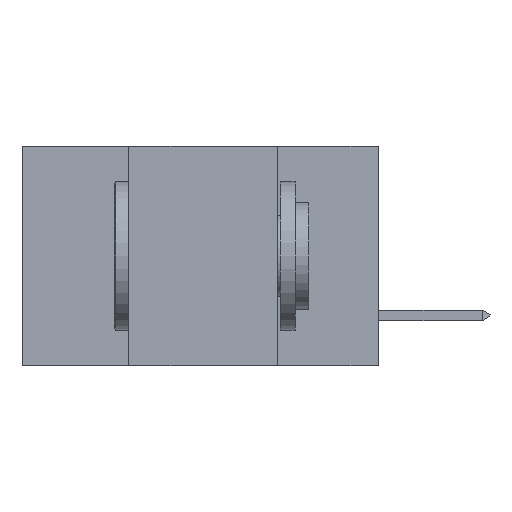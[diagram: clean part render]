
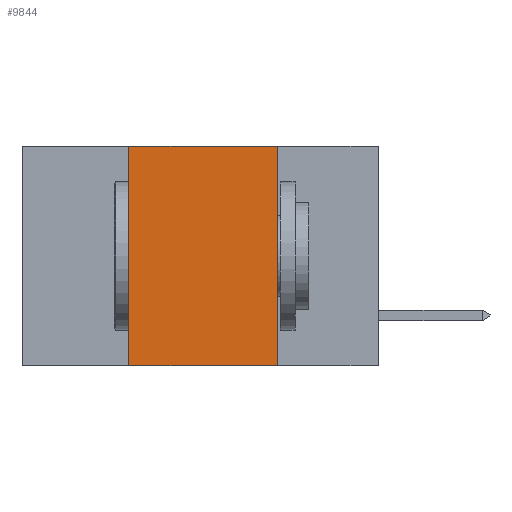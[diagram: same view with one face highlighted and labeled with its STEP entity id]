
A CAD part, left-side view. The second image highlights one B-rep face of the part: STEP entity #9844.
In plain terms, the highlighted planar face has unit normal (-1, 0, 0).
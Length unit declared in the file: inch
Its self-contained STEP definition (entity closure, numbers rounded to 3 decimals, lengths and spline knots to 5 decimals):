
#31 = EDGE_CURVE ( 'NONE', #1303, #6683, #638, .T. ) ;
#322 = LINE ( 'NONE', #10258, #9315 ) ;
#472 = ORIENTED_EDGE ( 'NONE', *, *, #728, .F. ) ;
#638 = LINE ( 'NONE', #683, #1599 ) ;
#683 = CARTESIAN_POINT ( 'NONE',  ( 0., 0.6, -0.37 ) ) ;
#699 = ORIENTED_EDGE ( 'NONE', *, *, #10522, .F. ) ;
#728 = EDGE_CURVE ( 'NONE', #3880, #6683, #9500, .T. ) ;
#843 = LINE ( 'NONE', #9961, #4532 ) ;
#1181 = DIRECTION ( 'NONE',  ( 0., -1., 0. ) ) ;
#1303 = VERTEX_POINT ( 'NONE', #3892 ) ;
#1599 = VECTOR ( 'NONE', #10632, 39.37008 ) ;
#1858 = DIRECTION ( 'NONE',  ( 0., 0., -1. ) ) ;
#2376 = CARTESIAN_POINT ( 'NONE',  ( 0., 0.17, 0. ) ) ;
#3576 = ORIENTED_EDGE ( 'NONE', *, *, #8541, .F. ) ;
#3579 = DIRECTION ( 'NONE',  ( 0., 0., -1. ) ) ;
#3880 = VERTEX_POINT ( 'NONE', #2376 ) ;
#3892 = CARTESIAN_POINT ( 'NONE',  ( 0., 0.42, -0.37 ) ) ;
#4230 = CARTESIAN_POINT ( 'NONE',  ( 0., 0.6, 0. ) ) ;
#4532 = VECTOR ( 'NONE', #5053, 39.37008 ) ;
#5053 = DIRECTION ( 'NONE',  ( 0., 0., 1. ) ) ;
#5348 = CARTESIAN_POINT ( 'NONE',  ( 0., 0.42, 0. ) ) ;
#6033 = CARTESIAN_POINT ( 'NONE',  ( 0., 0.17, -0.37 ) ) ;
#6683 = VERTEX_POINT ( 'NONE', #6033 ) ;
#6800 = VERTEX_POINT ( 'NONE', #5348 ) ;
#7447 = AXIS2_PLACEMENT_3D ( 'NONE', #4230, #8410, #1858 ) ;
#7848 = CARTESIAN_POINT ( 'NONE',  ( 0., 0.17, -0.37 ) ) ;
#8410 = DIRECTION ( 'NONE',  ( 1., 0., 0. ) ) ;
#8468 = PLANE ( 'NONE',  #7447 ) ;
#8541 = EDGE_CURVE ( 'NONE', #6800, #3880, #322, .T. ) ;
#8837 = ORIENTED_EDGE ( 'NONE', *, *, #31, .T. ) ;
#9104 = EDGE_LOOP ( 'NONE', ( #472, #3576, #699, #8837 ) ) ;
#9128 = FACE_OUTER_BOUND ( 'NONE', #9104, .T. ) ;
#9315 = VECTOR ( 'NONE', #1181, 39.37008 ) ;
#9500 = LINE ( 'NONE', #7848, #10221 ) ;
#9844 = ADVANCED_FACE ( 'NONE', ( #9128 ), #8468, .F. ) ;
#9961 = CARTESIAN_POINT ( 'NONE',  ( 0., 0.42, -0.37 ) ) ;
#10221 = VECTOR ( 'NONE', #3579, 39.37008 ) ;
#10258 = CARTESIAN_POINT ( 'NONE',  ( 0., 0.6, 0. ) ) ;
#10522 = EDGE_CURVE ( 'NONE', #1303, #6800, #843, .T. ) ;
#10632 = DIRECTION ( 'NONE',  ( 0., -1., 0. ) ) ;
